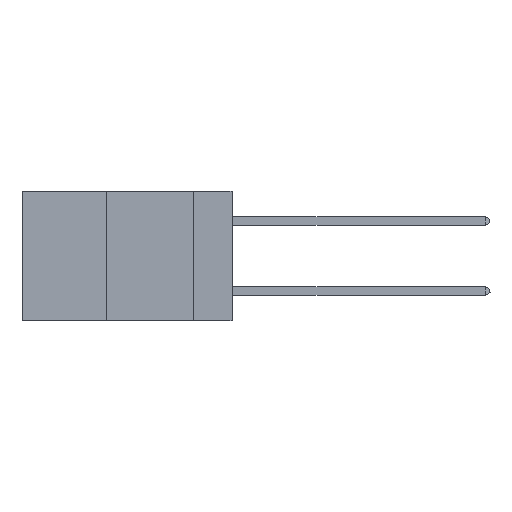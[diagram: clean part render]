
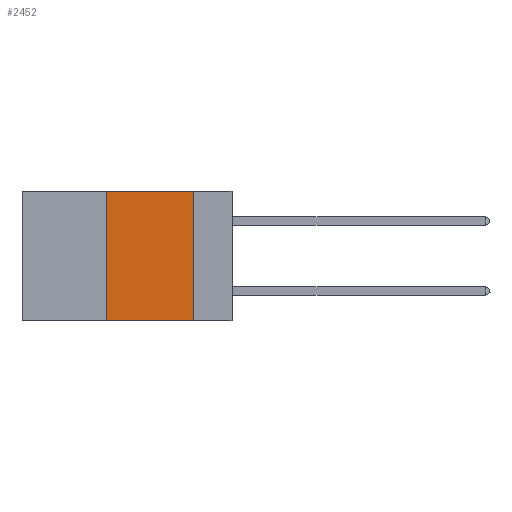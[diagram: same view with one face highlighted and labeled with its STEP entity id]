
A CAD part, left-side view. The second image highlights one B-rep face of the part: STEP entity #2452.
In plain terms, the highlighted planar face has unit normal (-1, 0, 0).
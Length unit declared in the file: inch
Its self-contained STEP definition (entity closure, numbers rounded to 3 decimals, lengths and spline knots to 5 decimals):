
#63 = PLANE ( 'NONE',  #5287 ) ;
#119 = CARTESIAN_POINT ( 'NONE',  ( 0., 0.6, 0. ) ) ;
#125 = LINE ( 'NONE', #5753, #17458 ) ;
#672 = LINE ( 'NONE', #15418, #10370 ) ;
#1042 = CARTESIAN_POINT ( 'NONE',  ( 0., 0.36, -0.37 ) ) ;
#1845 = EDGE_CURVE ( 'NONE', #13920, #16625, #8155, .T. ) ;
#2452 = ADVANCED_FACE ( 'NONE', ( #2463 ), #63, .F. ) ;
#2463 = FACE_OUTER_BOUND ( 'NONE', #5974, .T. ) ;
#2481 = LINE ( 'NONE', #4923, #7765 ) ;
#3319 = DIRECTION ( 'NONE',  ( 0., 0., 1. ) ) ;
#4051 = DIRECTION ( 'NONE',  ( 1., 0., 0. ) ) ;
#4168 = CARTESIAN_POINT ( 'NONE',  ( 0., 0.11, 0. ) ) ;
#4923 = CARTESIAN_POINT ( 'NONE',  ( 0., 0.11, 0. ) ) ;
#5287 = AXIS2_PLACEMENT_3D ( 'NONE', #119, #4051, #16333 ) ;
#5753 = CARTESIAN_POINT ( 'NONE',  ( 0., 0.6, 0. ) ) ;
#5974 = EDGE_LOOP ( 'NONE', ( #16718, #14876, #10682, #6178 ) ) ;
#6178 = ORIENTED_EDGE ( 'NONE', *, *, #1845, .T. ) ;
#7765 = VECTOR ( 'NONE', #11646, 39.37008 ) ;
#8155 = LINE ( 'NONE', #12310, #14709 ) ;
#8904 = EDGE_CURVE ( 'NONE', #14602, #10990, #125, .T. ) ;
#9963 = EDGE_CURVE ( 'NONE', #10990, #16625, #2481, .T. ) ;
#10370 = VECTOR ( 'NONE', #3319, 39.37008 ) ;
#10682 = ORIENTED_EDGE ( 'NONE', *, *, #12867, .F. ) ;
#10990 = VERTEX_POINT ( 'NONE', #4168 ) ;
#11646 = DIRECTION ( 'NONE',  ( 0., 0., -1. ) ) ;
#11793 = CARTESIAN_POINT ( 'NONE',  ( 0., 0.11, -0.37 ) ) ;
#12310 = CARTESIAN_POINT ( 'NONE',  ( 0., 0.6, -0.37 ) ) ;
#12867 = EDGE_CURVE ( 'NONE', #13920, #14602, #672, .T. ) ;
#13020 = CARTESIAN_POINT ( 'NONE',  ( 0., 0.36, 0. ) ) ;
#13920 = VERTEX_POINT ( 'NONE', #1042 ) ;
#14602 = VERTEX_POINT ( 'NONE', #13020 ) ;
#14709 = VECTOR ( 'NONE', #15002, 39.37008 ) ;
#14876 = ORIENTED_EDGE ( 'NONE', *, *, #8904, .F. ) ;
#15002 = DIRECTION ( 'NONE',  ( 0., -1., 0. ) ) ;
#15171 = DIRECTION ( 'NONE',  ( 0., -1., 0. ) ) ;
#15418 = CARTESIAN_POINT ( 'NONE',  ( 0., 0.36, 0. ) ) ;
#16333 = DIRECTION ( 'NONE',  ( 0., 0., -1. ) ) ;
#16625 = VERTEX_POINT ( 'NONE', #11793 ) ;
#16718 = ORIENTED_EDGE ( 'NONE', *, *, #9963, .F. ) ;
#17458 = VECTOR ( 'NONE', #15171, 39.37008 ) ;
